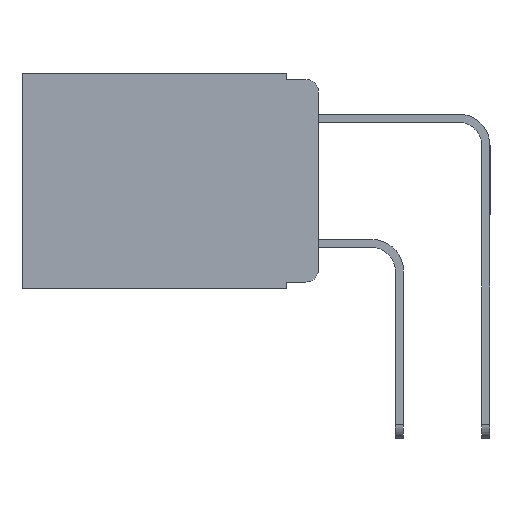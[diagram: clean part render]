
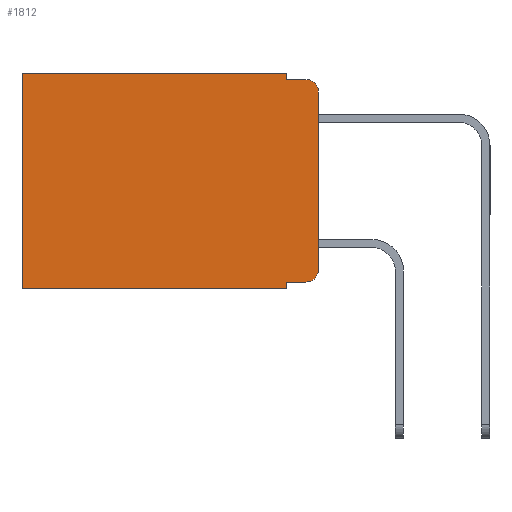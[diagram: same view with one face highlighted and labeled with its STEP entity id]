
A CAD part, left-side view. The second image highlights one B-rep face of the part: STEP entity #1812.
In plain terms, the highlighted planar face has unit normal (-1, 0, 0).
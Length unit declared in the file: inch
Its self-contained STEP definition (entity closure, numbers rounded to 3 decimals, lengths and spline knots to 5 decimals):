
#1275 = VERTEX_POINT ( 'NONE', #17679 ) ;
#1353 = VECTOR ( 'NONE', #17917, 39.37008 ) ;
#1390 = DIRECTION ( 'NONE',  ( 0., 0., -1. ) ) ;
#1812 = ADVANCED_FACE ( 'NONE', ( #8748 ), #17849, .F. ) ;
#2089 = EDGE_CURVE ( 'NONE', #9576, #12136, #17807, .T. ) ;
#2242 = CARTESIAN_POINT ( 'NONE',  ( 0.298, 0.051, 0. ) ) ;
#2805 = EDGE_CURVE ( 'NONE', #1275, #4987, #4189, .T. ) ;
#2860 = CARTESIAN_POINT ( 'NONE',  ( 0.298, 0., -0.343 ) ) ;
#3097 = VERTEX_POINT ( 'NONE', #15445 ) ;
#3311 = CARTESIAN_POINT ( 'NONE',  ( 0.298, 0.473, -0.343 ) ) ;
#3737 = ORIENTED_EDGE ( 'NONE', *, *, #21044, .T. ) ;
#3995 = VERTEX_POINT ( 'NONE', #19758 ) ;
#4049 = CARTESIAN_POINT ( 'NONE',  ( 0.298, 0.02, -0.313 ) ) ;
#4189 = LINE ( 'NONE', #2860, #20895 ) ;
#4303 = DIRECTION ( 'NONE',  ( 0., 0., -1. ) ) ;
#4418 = CARTESIAN_POINT ( 'NONE',  ( 0.298, 0.02, -0.03 ) ) ;
#4834 = ORIENTED_EDGE ( 'NONE', *, *, #2089, .F. ) ;
#4890 = LINE ( 'NONE', #12545, #13648 ) ;
#4987 = VERTEX_POINT ( 'NONE', #3311 ) ;
#5757 = DIRECTION ( 'NONE',  ( 0., 0., -1. ) ) ;
#6128 = DIRECTION ( 'NONE',  ( 0., 0., -1. ) ) ;
#6774 = AXIS2_PLACEMENT_3D ( 'NONE', #4418, #15901, #6128 ) ;
#7309 = LINE ( 'NONE', #2242, #7822 ) ;
#7336 = ORIENTED_EDGE ( 'NONE', *, *, #14715, .T. ) ;
#7602 = VERTEX_POINT ( 'NONE', #9689 ) ;
#7607 = VERTEX_POINT ( 'NONE', #19317 ) ;
#7822 = VECTOR ( 'NONE', #12226, 39.37008 ) ;
#8369 = DIRECTION ( 'NONE',  ( 0., -1., 0. ) ) ;
#8586 = ORIENTED_EDGE ( 'NONE', *, *, #2805, .F. ) ;
#8748 = FACE_OUTER_BOUND ( 'NONE', #10695, .T. ) ;
#8807 = DIRECTION ( 'NONE',  ( 0., -1., 0. ) ) ;
#8875 = VERTEX_POINT ( 'NONE', #19055 ) ;
#9366 = ORIENTED_EDGE ( 'NONE', *, *, #18996, .F. ) ;
#9576 = VERTEX_POINT ( 'NONE', #18828 ) ;
#9689 = CARTESIAN_POINT ( 'NONE',  ( 0.298, 0.02, -0.01 ) ) ;
#10132 = VECTOR ( 'NONE', #8369, 39.37008 ) ;
#10271 = LINE ( 'NONE', #19421, #1353 ) ;
#10351 = CARTESIAN_POINT ( 'NONE',  ( 0.298, 0., 0. ) ) ;
#10394 = CIRCLE ( 'NONE', #12760, 0.02 ) ;
#10644 = LINE ( 'NONE', #14797, #10132 ) ;
#10680 = DIRECTION ( 'NONE',  ( 0., 0., -1. ) ) ;
#10695 = EDGE_LOOP ( 'NONE', ( #4834, #3737, #19223, #9366, #13517, #20140, #8586, #13951, #14212, #7336 ) ) ;
#11414 = DIRECTION ( 'NONE',  ( 1., 0., 0. ) ) ;
#12136 = VERTEX_POINT ( 'NONE', #17580 ) ;
#12226 = DIRECTION ( 'NONE',  ( 0., 0., -1. ) ) ;
#12545 = CARTESIAN_POINT ( 'NONE',  ( 0.298, 0.473, 0. ) ) ;
#12672 = DIRECTION ( 'NONE',  ( 0., 1., 0. ) ) ;
#12760 = AXIS2_PLACEMENT_3D ( 'NONE', #4049, #15552, #5757 ) ;
#12973 = LINE ( 'NONE', #10351, #20890 ) ;
#13517 = ORIENTED_EDGE ( 'NONE', *, *, #14595, .T. ) ;
#13648 = VECTOR ( 'NONE', #4303, 39.37008 ) ;
#13652 = DIRECTION ( 'NONE',  ( 0., 1., 0. ) ) ;
#13791 = CARTESIAN_POINT ( 'NONE',  ( 0.298, 0.051, -0.01 ) ) ;
#13951 = ORIENTED_EDGE ( 'NONE', *, *, #16887, .F. ) ;
#14212 = ORIENTED_EDGE ( 'NONE', *, *, #15806, .T. ) ;
#14595 = EDGE_CURVE ( 'NONE', #7607, #8875, #12973, .T. ) ;
#14679 = VERTEX_POINT ( 'NONE', #13791 ) ;
#14715 = EDGE_CURVE ( 'NONE', #3995, #12136, #10394, .T. ) ;
#14797 = CARTESIAN_POINT ( 'NONE',  ( 0.298, 0.051, -0.333 ) ) ;
#15445 = CARTESIAN_POINT ( 'NONE',  ( 0.298, 0.051, -0.333 ) ) ;
#15552 = DIRECTION ( 'NONE',  ( -1., 0., 0. ) ) ;
#15596 = CARTESIAN_POINT ( 'NONE',  ( 0.298, 0., 0. ) ) ;
#15806 = EDGE_CURVE ( 'NONE', #3097, #3995, #10644, .T. ) ;
#15901 = DIRECTION ( 'NONE',  ( -1., 0., 0. ) ) ;
#16131 = LINE ( 'NONE', #20003, #16632 ) ;
#16632 = VECTOR ( 'NONE', #8807, 39.37008 ) ;
#16813 = VECTOR ( 'NONE', #10680, 39.37008 ) ;
#16887 = EDGE_CURVE ( 'NONE', #3097, #1275, #7309, .T. ) ;
#17580 = CARTESIAN_POINT ( 'NONE',  ( 0.298, 0., -0.313 ) ) ;
#17679 = CARTESIAN_POINT ( 'NONE',  ( 0.298, 0.051, -0.343 ) ) ;
#17807 = LINE ( 'NONE', #15596, #16813 ) ;
#17849 = PLANE ( 'NONE',  #18824 ) ;
#17917 = DIRECTION ( 'NONE',  ( 0., 0., -1. ) ) ;
#17941 = EDGE_CURVE ( 'NONE', #8875, #4987, #4890, .T. ) ;
#18824 = AXIS2_PLACEMENT_3D ( 'NONE', #20951, #11414, #1390 ) ;
#18828 = CARTESIAN_POINT ( 'NONE',  ( 0.298, 0., -0.03 ) ) ;
#18996 = EDGE_CURVE ( 'NONE', #7607, #14679, #10271, .T. ) ;
#19055 = CARTESIAN_POINT ( 'NONE',  ( 0.298, 0.473, 0. ) ) ;
#19223 = ORIENTED_EDGE ( 'NONE', *, *, #20039, .F. ) ;
#19317 = CARTESIAN_POINT ( 'NONE',  ( 0.298, 0.051, 0. ) ) ;
#19421 = CARTESIAN_POINT ( 'NONE',  ( 0.298, 0.051, 0. ) ) ;
#19758 = CARTESIAN_POINT ( 'NONE',  ( 0.298, 0.02, -0.333 ) ) ;
#20003 = CARTESIAN_POINT ( 'NONE',  ( 0.298, 0.051, -0.01 ) ) ;
#20039 = EDGE_CURVE ( 'NONE', #14679, #7602, #16131, .T. ) ;
#20140 = ORIENTED_EDGE ( 'NONE', *, *, #17941, .T. ) ;
#20890 = VECTOR ( 'NONE', #13652, 39.37008 ) ;
#20895 = VECTOR ( 'NONE', #12672, 39.37008 ) ;
#20951 = CARTESIAN_POINT ( 'NONE',  ( 0.298, 0., 0. ) ) ;
#21044 = EDGE_CURVE ( 'NONE', #9576, #7602, #21218, .T. ) ;
#21218 = CIRCLE ( 'NONE', #6774, 0.02 ) ;
